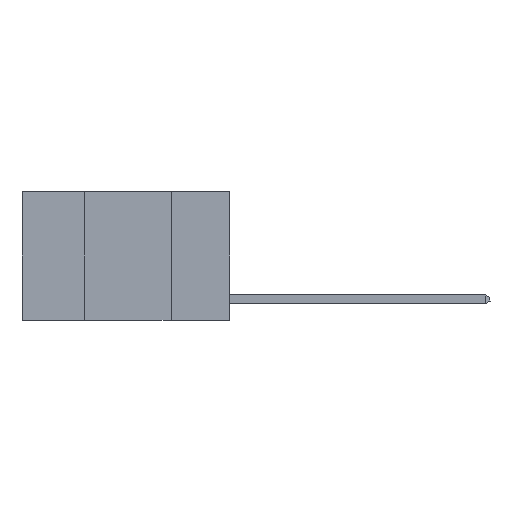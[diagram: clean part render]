
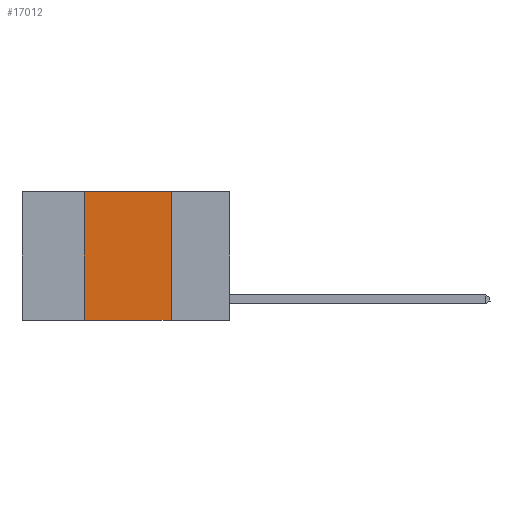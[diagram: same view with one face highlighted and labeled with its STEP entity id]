
A CAD part, left-side view. The second image highlights one B-rep face of the part: STEP entity #17012.
In plain terms, the highlighted planar face has unit normal (-1, 0, 0).
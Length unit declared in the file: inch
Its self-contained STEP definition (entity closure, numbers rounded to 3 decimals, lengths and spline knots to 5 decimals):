
#565 = EDGE_CURVE ( 'NONE', #6746, #20316, #17939, .T. ) ;
#652 = LINE ( 'NONE', #5944, #21455 ) ;
#1238 = DIRECTION ( 'NONE',  ( 0., 0., -1. ) ) ;
#1574 = CARTESIAN_POINT ( 'NONE',  ( 0., 0.6, 0. ) ) ;
#2535 = DIRECTION ( 'NONE',  ( 0., -1., 0. ) ) ;
#3447 = CARTESIAN_POINT ( 'NONE',  ( 0., 0.17, 0. ) ) ;
#5139 = VECTOR ( 'NONE', #2535, 39.37008 ) ;
#5944 = CARTESIAN_POINT ( 'NONE',  ( 0., 0.17, 0. ) ) ;
#6575 = VERTEX_POINT ( 'NONE', #3447 ) ;
#6746 = VERTEX_POINT ( 'NONE', #10877 ) ;
#7199 = LINE ( 'NONE', #12495, #19607 ) ;
#8654 = CARTESIAN_POINT ( 'NONE',  ( 0., 0.17, -0.37 ) ) ;
#9063 = VERTEX_POINT ( 'NONE', #8654 ) ;
#10877 = CARTESIAN_POINT ( 'NONE',  ( 0., 0.42, -0.37 ) ) ;
#11511 = EDGE_LOOP ( 'NONE', ( #16042, #12863, #17025, #14798 ) ) ;
#11604 = FACE_OUTER_BOUND ( 'NONE', #11511, .T. ) ;
#11933 = PLANE ( 'NONE',  #13112 ) ;
#12495 = CARTESIAN_POINT ( 'NONE',  ( 0., 0.6, -0.37 ) ) ;
#12863 = ORIENTED_EDGE ( 'NONE', *, *, #13015, .F. ) ;
#13015 = EDGE_CURVE ( 'NONE', #20316, #6575, #14785, .T. ) ;
#13112 = AXIS2_PLACEMENT_3D ( 'NONE', #1574, #22085, #1238 ) ;
#14075 = DIRECTION ( 'NONE',  ( 0., -1., 0. ) ) ;
#14785 = LINE ( 'NONE', #16476, #5139 ) ;
#14798 = ORIENTED_EDGE ( 'NONE', *, *, #15021, .T. ) ;
#15021 = EDGE_CURVE ( 'NONE', #6746, #9063, #7199, .T. ) ;
#16042 = ORIENTED_EDGE ( 'NONE', *, *, #19063, .F. ) ;
#16242 = CARTESIAN_POINT ( 'NONE',  ( 0., 0.42, 0. ) ) ;
#16476 = CARTESIAN_POINT ( 'NONE',  ( 0., 0.6, 0. ) ) ;
#17012 = ADVANCED_FACE ( 'NONE', ( #11604 ), #11933, .F. ) ;
#17025 = ORIENTED_EDGE ( 'NONE', *, *, #565, .F. ) ;
#17939 = LINE ( 'NONE', #16242, #21525 ) ;
#19063 = EDGE_CURVE ( 'NONE', #6575, #9063, #652, .T. ) ;
#19607 = VECTOR ( 'NONE', #14075, 39.37008 ) ;
#19900 = DIRECTION ( 'NONE',  ( 0., 0., -1. ) ) ;
#20316 = VERTEX_POINT ( 'NONE', #21190 ) ;
#21190 = CARTESIAN_POINT ( 'NONE',  ( 0., 0.42, 0. ) ) ;
#21455 = VECTOR ( 'NONE', #19900, 39.37008 ) ;
#21525 = VECTOR ( 'NONE', #21860, 39.37008 ) ;
#21860 = DIRECTION ( 'NONE',  ( 0., 0., 1. ) ) ;
#22085 = DIRECTION ( 'NONE',  ( 1., 0., 0. ) ) ;
